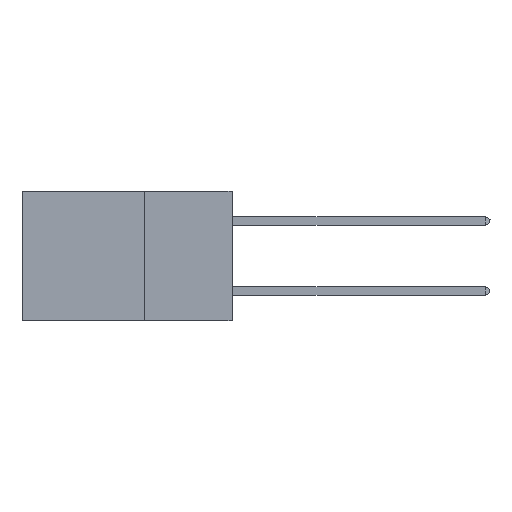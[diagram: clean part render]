
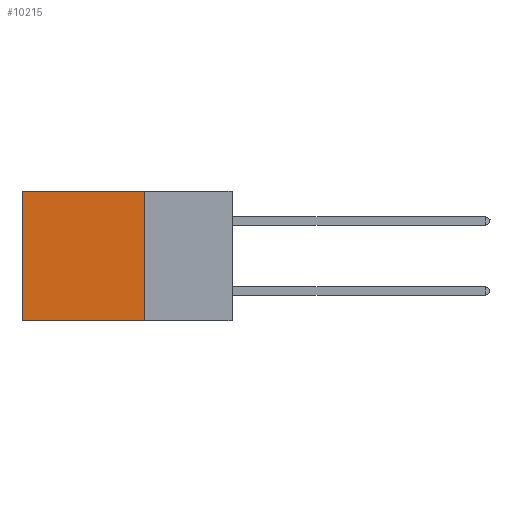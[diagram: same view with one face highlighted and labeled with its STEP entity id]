
A CAD part, left-side view. The second image highlights one B-rep face of the part: STEP entity #10215.
In plain terms, the highlighted planar face has unit normal (-1, 0, 0).
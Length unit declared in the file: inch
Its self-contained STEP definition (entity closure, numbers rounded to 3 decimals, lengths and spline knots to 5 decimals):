
#385 = ORIENTED_EDGE ( 'NONE', *, *, #34025, .F. ) ;
#850 = VERTEX_POINT ( 'NONE', #36998 ) ;
#3544 = DIRECTION ( 'NONE',  ( 0., 1., 0. ) ) ;
#4598 = CARTESIAN_POINT ( 'NONE',  ( 0.2875, 0.6, 0. ) ) ;
#4738 = CARTESIAN_POINT ( 'NONE',  ( 0.2875, 0.25, -0.37 ) ) ;
#4996 = PLANE ( 'NONE',  #13620 ) ;
#6816 = EDGE_CURVE ( 'NONE', #33816, #36550, #11017, .T. ) ;
#8132 = CARTESIAN_POINT ( 'NONE',  ( 0.2875, 0.25, 0. ) ) ;
#8579 = LINE ( 'NONE', #32032, #8883 ) ;
#8883 = VECTOR ( 'NONE', #14276, 39.37008 ) ;
#10215 = ADVANCED_FACE ( 'NONE', ( #14400 ), #4996, .F. ) ;
#11017 = LINE ( 'NONE', #4738, #34088 ) ;
#11469 = ORIENTED_EDGE ( 'NONE', *, *, #19243, .T. ) ;
#11891 = VERTEX_POINT ( 'NONE', #36650 ) ;
#13429 = LINE ( 'NONE', #4598, #36575 ) ;
#13620 = AXIS2_PLACEMENT_3D ( 'NONE', #8132, #31573, #22587 ) ;
#14276 = DIRECTION ( 'NONE',  ( 0., 0., -1. ) ) ;
#14400 = FACE_OUTER_BOUND ( 'NONE', #37624, .T. ) ;
#15684 = LINE ( 'NONE', #21915, #18306 ) ;
#18306 = VECTOR ( 'NONE', #3544, 39.37008 ) ;
#19087 = DIRECTION ( 'NONE',  ( 0., 0., -1. ) ) ;
#19243 = EDGE_CURVE ( 'NONE', #850, #11891, #15684, .T. ) ;
#21915 = CARTESIAN_POINT ( 'NONE',  ( 0.2875, 0.25, 0. ) ) ;
#22101 = EDGE_CURVE ( 'NONE', #11891, #36550, #13429, .T. ) ;
#22587 = DIRECTION ( 'NONE',  ( 0., 0., -1. ) ) ;
#25417 = ORIENTED_EDGE ( 'NONE', *, *, #6816, .F. ) ;
#25657 = DIRECTION ( 'NONE',  ( 0., 1., 0. ) ) ;
#29088 = ORIENTED_EDGE ( 'NONE', *, *, #22101, .T. ) ;
#31573 = DIRECTION ( 'NONE',  ( 1., 0., 0. ) ) ;
#32032 = CARTESIAN_POINT ( 'NONE',  ( 0.2875, 0.25, 0. ) ) ;
#33816 = VERTEX_POINT ( 'NONE', #35038 ) ;
#34025 = EDGE_CURVE ( 'NONE', #850, #33816, #8579, .T. ) ;
#34088 = VECTOR ( 'NONE', #25657, 39.37008 ) ;
#35038 = CARTESIAN_POINT ( 'NONE',  ( 0.2875, 0.25, -0.37 ) ) ;
#36550 = VERTEX_POINT ( 'NONE', #36757 ) ;
#36575 = VECTOR ( 'NONE', #19087, 39.37008 ) ;
#36650 = CARTESIAN_POINT ( 'NONE',  ( 0.2875, 0.6, 0. ) ) ;
#36757 = CARTESIAN_POINT ( 'NONE',  ( 0.2875, 0.6, -0.37 ) ) ;
#36998 = CARTESIAN_POINT ( 'NONE',  ( 0.2875, 0.25, 0. ) ) ;
#37624 = EDGE_LOOP ( 'NONE', ( #29088, #25417, #385, #11469 ) ) ;
